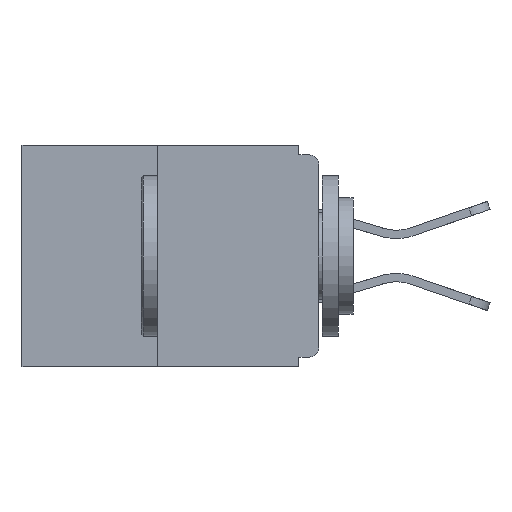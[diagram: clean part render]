
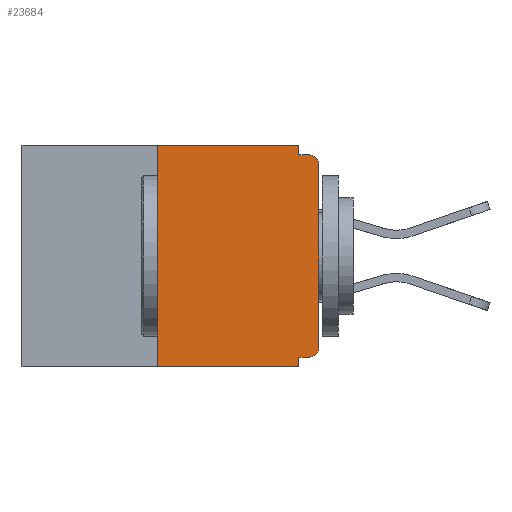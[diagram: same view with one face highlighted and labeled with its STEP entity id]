
A CAD part, left-side view. The second image highlights one B-rep face of the part: STEP entity #23684.
In plain terms, the highlighted planar face has unit normal (-1, 0, 0).
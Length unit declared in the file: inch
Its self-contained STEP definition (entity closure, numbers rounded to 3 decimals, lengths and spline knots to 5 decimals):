
#98 = LINE ( 'NONE', #6738, #22224 ) ;
#110 = CARTESIAN_POINT ( 'NONE',  ( 0., 0.25, 0. ) ) ;
#283 = CARTESIAN_POINT ( 'NONE',  ( 0., 0.031, 0. ) ) ;
#550 = LINE ( 'NONE', #22068, #16555 ) ;
#1070 = VECTOR ( 'NONE', #25457, 39.37008 ) ;
#1072 = VERTEX_POINT ( 'NONE', #5308 ) ;
#1311 = AXIS2_PLACEMENT_3D ( 'NONE', #6371, #25003, #14778 ) ;
#1988 = VERTEX_POINT ( 'NONE', #4775 ) ;
#2332 = CARTESIAN_POINT ( 'NONE',  ( 0., 0., 0. ) ) ;
#2844 = EDGE_CURVE ( 'NONE', #7240, #9856, #23290, .T. ) ;
#2861 = CIRCLE ( 'NONE', #1311, 0.015 ) ;
#3183 = VERTEX_POINT ( 'NONE', #20234 ) ;
#3370 = LINE ( 'NONE', #9462, #18076 ) ;
#3520 = EDGE_CURVE ( 'NONE', #16512, #1072, #22602, .T. ) ;
#3533 = LINE ( 'NONE', #110, #10432 ) ;
#3754 = DIRECTION ( 'NONE',  ( 0., 0., -1. ) ) ;
#3838 = VECTOR ( 'NONE', #16944, 39.37008 ) ;
#3970 = FACE_OUTER_BOUND ( 'NONE', #19021, .T. ) ;
#4051 = ORIENTED_EDGE ( 'NONE', *, *, #20725, .F. ) ;
#4369 = VECTOR ( 'NONE', #15048, 39.37008 ) ;
#4758 = CARTESIAN_POINT ( 'NONE',  ( 0., 0., -0.328 ) ) ;
#4775 = CARTESIAN_POINT ( 'NONE',  ( 0., 0., -0.03 ) ) ;
#4895 = ORIENTED_EDGE ( 'NONE', *, *, #2844, .F. ) ;
#4940 = CARTESIAN_POINT ( 'NONE',  ( 0., 0.031, -0.015 ) ) ;
#5136 = CIRCLE ( 'NONE', #13519, 0.015 ) ;
#5308 = CARTESIAN_POINT ( 'NONE',  ( 0., 0.031, -0.328 ) ) ;
#5383 = CARTESIAN_POINT ( 'NONE',  ( 0., 0.46, 0. ) ) ;
#6224 = EDGE_CURVE ( 'NONE', #20370, #1988, #21465, .T. ) ;
#6371 = CARTESIAN_POINT ( 'NONE',  ( 0., 0.015, -0.313 ) ) ;
#6380 = VECTOR ( 'NONE', #7673, 39.37008 ) ;
#6738 = CARTESIAN_POINT ( 'NONE',  ( 0., 0., -0.015 ) ) ;
#7240 = VERTEX_POINT ( 'NONE', #283 ) ;
#7648 = ORIENTED_EDGE ( 'NONE', *, *, #12223, .F. ) ;
#7673 = DIRECTION ( 'NONE',  ( 0., -1., 0. ) ) ;
#8680 = VERTEX_POINT ( 'NONE', #20309 ) ;
#9423 = EDGE_CURVE ( 'NONE', #1988, #3183, #5136, .T. ) ;
#9458 = ORIENTED_EDGE ( 'NONE', *, *, #18918, .T. ) ;
#9462 = CARTESIAN_POINT ( 'NONE',  ( 0., 0.031, -0.343 ) ) ;
#9856 = VERTEX_POINT ( 'NONE', #4940 ) ;
#9935 = AXIS2_PLACEMENT_3D ( 'NONE', #26898, #16174, #22319 ) ;
#10432 = VECTOR ( 'NONE', #25416, 39.37008 ) ;
#12223 = EDGE_CURVE ( 'NONE', #1072, #24644, #3370, .T. ) ;
#12571 = CARTESIAN_POINT ( 'NONE',  ( 0., 0., -0.313 ) ) ;
#13348 = EDGE_CURVE ( 'NONE', #9856, #3183, #98, .T. ) ;
#13519 = AXIS2_PLACEMENT_3D ( 'NONE', #18293, #18096, #3754 ) ;
#14508 = ORIENTED_EDGE ( 'NONE', *, *, #19457, .T. ) ;
#14778 = DIRECTION ( 'NONE',  ( 0., 0., -1. ) ) ;
#15048 = DIRECTION ( 'NONE',  ( 0., 0., -1. ) ) ;
#16174 = DIRECTION ( 'NONE',  ( 1., 0., 0. ) ) ;
#16354 = VERTEX_POINT ( 'NONE', #17620 ) ;
#16512 = VERTEX_POINT ( 'NONE', #22041 ) ;
#16555 = VECTOR ( 'NONE', #26543, 39.37008 ) ;
#16858 = LINE ( 'NONE', #5383, #6380 ) ;
#16942 = ORIENTED_EDGE ( 'NONE', *, *, #26235, .F. ) ;
#16944 = DIRECTION ( 'NONE',  ( 0., 0., 1. ) ) ;
#17620 = CARTESIAN_POINT ( 'NONE',  ( 0., 0.25, -0.343 ) ) ;
#17981 = ORIENTED_EDGE ( 'NONE', *, *, #3520, .F. ) ;
#18076 = VECTOR ( 'NONE', #24051, 39.37008 ) ;
#18096 = DIRECTION ( 'NONE',  ( -1., 0., 0. ) ) ;
#18293 = CARTESIAN_POINT ( 'NONE',  ( 0., 0.015, -0.03 ) ) ;
#18918 = EDGE_CURVE ( 'NONE', #16512, #20370, #2861, .T. ) ;
#19021 = EDGE_LOOP ( 'NONE', ( #4051, #16942, #14508, #7648, #17981, #9458, #20729, #26225, #26940, #4895 ) ) ;
#19338 = DIRECTION ( 'NONE',  ( 0., -1., 0. ) ) ;
#19457 = EDGE_CURVE ( 'NONE', #16354, #24644, #550, .T. ) ;
#20234 = CARTESIAN_POINT ( 'NONE',  ( 0., 0.015, -0.015 ) ) ;
#20309 = CARTESIAN_POINT ( 'NONE',  ( 0., 0.25, 0. ) ) ;
#20370 = VERTEX_POINT ( 'NONE', #12571 ) ;
#20725 = EDGE_CURVE ( 'NONE', #8680, #7240, #16858, .T. ) ;
#20729 = ORIENTED_EDGE ( 'NONE', *, *, #6224, .T. ) ;
#21465 = LINE ( 'NONE', #2332, #3838 ) ;
#21592 = CARTESIAN_POINT ( 'NONE',  ( 0., 0.031, 0. ) ) ;
#21812 = CARTESIAN_POINT ( 'NONE',  ( 0., 0.031, -0.343 ) ) ;
#22041 = CARTESIAN_POINT ( 'NONE',  ( 0., 0.015, -0.328 ) ) ;
#22068 = CARTESIAN_POINT ( 'NONE',  ( 0., 0.46, -0.343 ) ) ;
#22224 = VECTOR ( 'NONE', #19338, 39.37008 ) ;
#22319 = DIRECTION ( 'NONE',  ( 0., 0., -1. ) ) ;
#22417 = PLANE ( 'NONE',  #9935 ) ;
#22602 = LINE ( 'NONE', #4758, #1070 ) ;
#23290 = LINE ( 'NONE', #21592, #4369 ) ;
#23684 = ADVANCED_FACE ( 'NONE', ( #3970 ), #22417, .F. ) ;
#24051 = DIRECTION ( 'NONE',  ( 0., 0., -1. ) ) ;
#24644 = VERTEX_POINT ( 'NONE', #21812 ) ;
#25003 = DIRECTION ( 'NONE',  ( -1., 0., 0. ) ) ;
#25416 = DIRECTION ( 'NONE',  ( 0., 0., 1. ) ) ;
#25457 = DIRECTION ( 'NONE',  ( 0., 1., 0. ) ) ;
#26225 = ORIENTED_EDGE ( 'NONE', *, *, #9423, .T. ) ;
#26235 = EDGE_CURVE ( 'NONE', #16354, #8680, #3533, .T. ) ;
#26543 = DIRECTION ( 'NONE',  ( 0., -1., 0. ) ) ;
#26898 = CARTESIAN_POINT ( 'NONE',  ( 0., 0.46, 0. ) ) ;
#26940 = ORIENTED_EDGE ( 'NONE', *, *, #13348, .F. ) ;
